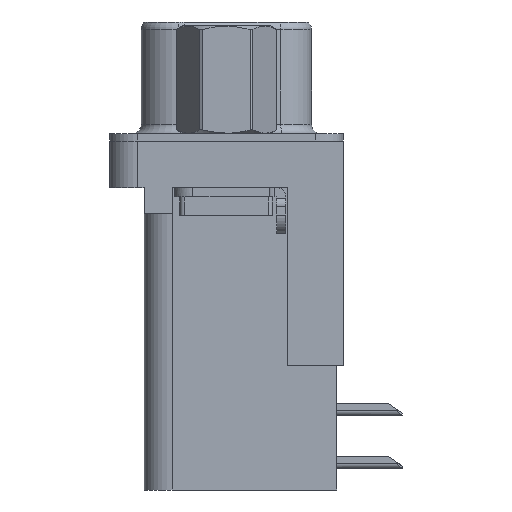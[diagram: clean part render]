
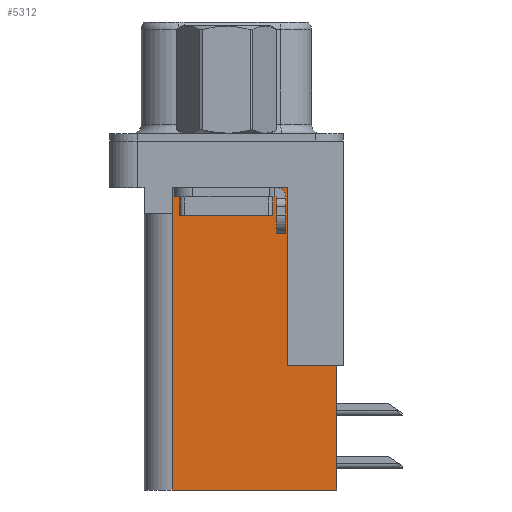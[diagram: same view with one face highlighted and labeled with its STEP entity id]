
A CAD part, left-side view. The second image highlights one B-rep face of the part: STEP entity #5312.
In plain terms, the highlighted planar face has unit normal (-1, 0, 0).
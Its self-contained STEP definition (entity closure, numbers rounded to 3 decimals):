
#122 = VERTEX_POINT ( 'NONE', #12038 ) ;
#232 = VECTOR ( 'NONE', #3830, 1000. ) ;
#289 = DIRECTION ( 'NONE',  ( 0., 1., 0. ) ) ;
#392 = CARTESIAN_POINT ( 'NONE',  ( 3.79, -6.295, -12.05 ) ) ;
#641 = VERTEX_POINT ( 'NONE', #11904 ) ;
#1071 = VERTEX_POINT ( 'NONE', #20906 ) ;
#1765 = PLANE ( 'NONE',  #6119 ) ;
#1842 = DIRECTION ( 'NONE',  ( 1., 0., 0. ) ) ;
#2005 = CARTESIAN_POINT ( 'NONE',  ( 3.79, -3.295, -2.5 ) ) ;
#2145 = VERTEX_POINT ( 'NONE', #4097 ) ;
#2336 = EDGE_CURVE ( 'NONE', #641, #16720, #17434, .T. ) ;
#2607 = VECTOR ( 'NONE', #7951, 1000. ) ;
#2650 = LINE ( 'NONE', #2937, #6983 ) ;
#2782 = EDGE_CURVE ( 'NONE', #16720, #2145, #15627, .T. ) ;
#2937 = CARTESIAN_POINT ( 'NONE',  ( 3.79, 2.925, -18.76 ) ) ;
#3338 = VECTOR ( 'NONE', #20993, 1000. ) ;
#3397 = ORIENTED_EDGE ( 'NONE', *, *, #4166, .T. ) ;
#3559 = VECTOR ( 'NONE', #289, 1000. ) ;
#3830 = DIRECTION ( 'NONE',  ( 0., 1., 0. ) ) ;
#3906 = CARTESIAN_POINT ( 'NONE',  ( 3.79, 2.895, -3.9 ) ) ;
#4032 = EDGE_CURVE ( 'NONE', #122, #1071, #6675, .T. ) ;
#4083 = VERTEX_POINT ( 'NONE', #21156 ) ;
#4097 = CARTESIAN_POINT ( 'NONE',  ( 3.79, 2.925, -3.9 ) ) ;
#4166 = EDGE_CURVE ( 'NONE', #4083, #122, #13332, .T. ) ;
#4186 = CARTESIAN_POINT ( 'NONE',  ( 3.79, 2.895, -3.9 ) ) ;
#4379 = VECTOR ( 'NONE', #6848, 1000. ) ;
#4825 = EDGE_CURVE ( 'NONE', #4083, #18351, #8455, .T. ) ;
#4859 = EDGE_CURVE ( 'NONE', #18351, #9559, #7914, .T. ) ;
#5312 = ADVANCED_FACE ( 'NONE', ( #5593 ), #1765, .F. ) ;
#5593 = FACE_OUTER_BOUND ( 'NONE', #7024, .T. ) ;
#5731 = EDGE_CURVE ( 'NONE', #9559, #2145, #2650, .T. ) ;
#6119 = AXIS2_PLACEMENT_3D ( 'NONE', #8316, #1842, #13242 ) ;
#6675 = LINE ( 'NONE', #7393, #3338 ) ;
#6848 = DIRECTION ( 'NONE',  ( 0., 0., -1. ) ) ;
#6983 = VECTOR ( 'NONE', #16019, 1000. ) ;
#7024 = EDGE_LOOP ( 'NONE', ( #12873, #19493, #11747, #18698, #19764, #16349, #3397, #11974 ) ) ;
#7393 = CARTESIAN_POINT ( 'NONE',  ( 3.79, -3.295, -18.76 ) ) ;
#7511 = LINE ( 'NONE', #2005, #16238 ) ;
#7801 = CARTESIAN_POINT ( 'NONE',  ( 3.79, 0., -3.9 ) ) ;
#7914 = LINE ( 'NONE', #8490, #3559 ) ;
#7951 = DIRECTION ( 'NONE',  ( 0., 1., 0. ) ) ;
#8316 = CARTESIAN_POINT ( 'NONE',  ( 3.79, -3.295, -18.76 ) ) ;
#8455 = LINE ( 'NONE', #16625, #17139 ) ;
#8490 = CARTESIAN_POINT ( 'NONE',  ( 3.79, -3.295, -18.76 ) ) ;
#9398 = CARTESIAN_POINT ( 'NONE',  ( 3.79, -5.925, -18.76 ) ) ;
#9559 = VERTEX_POINT ( 'NONE', #11446 ) ;
#11446 = CARTESIAN_POINT ( 'NONE',  ( 3.79, 2.925, -18.76 ) ) ;
#11747 = ORIENTED_EDGE ( 'NONE', *, *, #2782, .T. ) ;
#11758 = DIRECTION ( 'NONE',  ( 0., 1., 0. ) ) ;
#11904 = CARTESIAN_POINT ( 'NONE',  ( 3.79, 2.895, -2.5 ) ) ;
#11974 = ORIENTED_EDGE ( 'NONE', *, *, #4032, .T. ) ;
#12038 = CARTESIAN_POINT ( 'NONE',  ( 3.79, -3.295, -12.05 ) ) ;
#12873 = ORIENTED_EDGE ( 'NONE', *, *, #21008, .T. ) ;
#13242 = DIRECTION ( 'NONE',  ( 0., 1., 0. ) ) ;
#13332 = LINE ( 'NONE', #392, #232 ) ;
#13346 = DIRECTION ( 'NONE',  ( 0., 0., -1. ) ) ;
#15627 = LINE ( 'NONE', #7801, #2607 ) ;
#16019 = DIRECTION ( 'NONE',  ( 0., 0., 1. ) ) ;
#16238 = VECTOR ( 'NONE', #11758, 1000. ) ;
#16349 = ORIENTED_EDGE ( 'NONE', *, *, #4825, .F. ) ;
#16625 = CARTESIAN_POINT ( 'NONE',  ( 3.79, -5.925, -2. ) ) ;
#16720 = VERTEX_POINT ( 'NONE', #3906 ) ;
#17139 = VECTOR ( 'NONE', #13346, 1000. ) ;
#17434 = LINE ( 'NONE', #4186, #4379 ) ;
#18351 = VERTEX_POINT ( 'NONE', #9398 ) ;
#18698 = ORIENTED_EDGE ( 'NONE', *, *, #5731, .F. ) ;
#19493 = ORIENTED_EDGE ( 'NONE', *, *, #2336, .T. ) ;
#19764 = ORIENTED_EDGE ( 'NONE', *, *, #4859, .F. ) ;
#20906 = CARTESIAN_POINT ( 'NONE',  ( 3.79, -3.295, -2.5 ) ) ;
#20993 = DIRECTION ( 'NONE',  ( 0., 0., 1. ) ) ;
#21008 = EDGE_CURVE ( 'NONE', #1071, #641, #7511, .T. ) ;
#21156 = CARTESIAN_POINT ( 'NONE',  ( 3.79, -5.925, -12.05 ) ) ;
